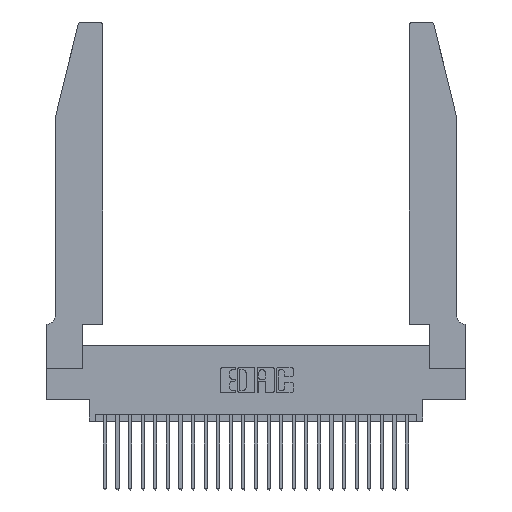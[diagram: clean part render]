
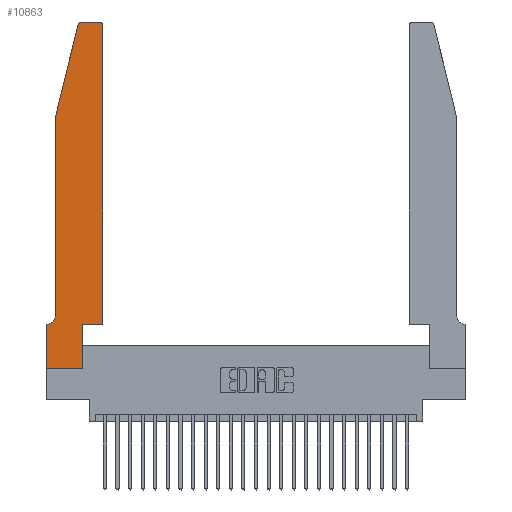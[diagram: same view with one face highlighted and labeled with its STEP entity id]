
A CAD part, top view. The second image highlights one B-rep face of the part: STEP entity #10863.
In plain terms, the highlighted planar face has unit normal (0, 0, 1).
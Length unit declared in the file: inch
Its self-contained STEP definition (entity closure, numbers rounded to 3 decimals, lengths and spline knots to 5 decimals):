
#157 = VERTEX_POINT ( 'NONE', #16407 ) ;
#285 = VECTOR ( 'NONE', #8463, 39.37008 ) ;
#910 = CIRCLE ( 'NONE', #12927, 0.03 ) ;
#916 = VERTEX_POINT ( 'NONE', #26282 ) ;
#1089 = LINE ( 'NONE', #9641, #23733 ) ;
#1887 = EDGE_CURVE ( 'NONE', #157, #13889, #9373, .T. ) ;
#2036 = VERTEX_POINT ( 'NONE', #17268 ) ;
#2094 = CARTESIAN_POINT ( 'NONE',  ( 0.284, 2.72, 0.37 ) ) ;
#2252 = CARTESIAN_POINT ( 'NONE',  ( 0.2865, 0.35, 0.37 ) ) ;
#2942 = ORIENTED_EDGE ( 'NONE', *, *, #4975, .T. ) ;
#3095 = CARTESIAN_POINT ( 'NONE',  ( 0.2605, 2.75, 0.37 ) ) ;
#3491 = CARTESIAN_POINT ( 'NONE',  ( 0.0755, 2., 0.37 ) ) ;
#3635 = ORIENTED_EDGE ( 'NONE', *, *, #1887, .T. ) ;
#3643 = CARTESIAN_POINT ( 'NONE',  ( 0.2865, 0.35, 0.37 ) ) ;
#3663 = VECTOR ( 'NONE', #6181, 39.37008 ) ;
#3993 = VERTEX_POINT ( 'NONE', #17073 ) ;
#4224 = CARTESIAN_POINT ( 'NONE',  ( 0., 0., 0.37 ) ) ;
#4352 = EDGE_CURVE ( 'NONE', #10704, #9987, #6673, .T. ) ;
#4615 = VERTEX_POINT ( 'NONE', #3491 ) ;
#4753 = DIRECTION ( 'NONE',  ( 1., 0., 0. ) ) ;
#4808 = DIRECTION ( 'NONE',  ( 1., 0., 0. ) ) ;
#4975 = EDGE_CURVE ( 'NONE', #25840, #17208, #22761, .T. ) ;
#5044 = VECTOR ( 'NONE', #5549, 39.37008 ) ;
#5361 = ORIENTED_EDGE ( 'NONE', *, *, #22117, .T. ) ;
#5549 = DIRECTION ( 'NONE',  ( 0., -1., 0. ) ) ;
#6181 = DIRECTION ( 'NONE',  ( 0., 1., 0. ) ) ;
#6673 = LINE ( 'NONE', #3095, #12470 ) ;
#7152 = LINE ( 'NONE', #15233, #22355 ) ;
#7387 = DIRECTION ( 'NONE',  ( -1., 0., 0. ) ) ;
#7452 = DIRECTION ( 'NONE',  ( -1., 0., 0. ) ) ;
#7631 = VECTOR ( 'NONE', #16535, 39.37008 ) ;
#7964 = CIRCLE ( 'NONE', #21372, 0.03 ) ;
#8151 = DIRECTION ( 'NONE',  ( -0.239, -0.971, 0. ) ) ;
#8463 = DIRECTION ( 'NONE',  ( 0., 1., 0. ) ) ;
#8710 = CARTESIAN_POINT ( 'NONE',  ( 0.4505, 2.72, 0.37 ) ) ;
#9137 = EDGE_CURVE ( 'NONE', #3993, #157, #12475, .T. ) ;
#9197 = ORIENTED_EDGE ( 'NONE', *, *, #24681, .T. ) ;
#9373 = LINE ( 'NONE', #2252, #285 ) ;
#9641 = CARTESIAN_POINT ( 'NONE',  ( 0.0755, 0.35, 0.37 ) ) ;
#9942 = CARTESIAN_POINT ( 'NONE',  ( 0.284, 2.75, 0.37 ) ) ;
#9987 = VERTEX_POINT ( 'NONE', #9942 ) ;
#10704 = VERTEX_POINT ( 'NONE', #20149 ) ;
#10863 = ADVANCED_FACE ( 'NONE', ( #24377 ), #24556, .T. ) ;
#11103 = ORIENTED_EDGE ( 'NONE', *, *, #12768, .T. ) ;
#11182 = VECTOR ( 'NONE', #4753, 39.37008 ) ;
#12092 = VECTOR ( 'NONE', #8151, 39.37008 ) ;
#12470 = VECTOR ( 'NONE', #7452, 39.37008 ) ;
#12475 = LINE ( 'NONE', #4224, #7631 ) ;
#12737 = LINE ( 'NONE', #14265, #12092 ) ;
#12768 = EDGE_CURVE ( 'NONE', #13889, #25840, #21846, .T. ) ;
#12797 = DIRECTION ( 'NONE',  ( 0., 0., -1. ) ) ;
#12927 = AXIS2_PLACEMENT_3D ( 'NONE', #2094, #18636, #26646 ) ;
#12943 = EDGE_CURVE ( 'NONE', #17208, #10704, #7964, .T. ) ;
#13015 = EDGE_CURVE ( 'NONE', #13371, #916, #1089, .T. ) ;
#13371 = VERTEX_POINT ( 'NONE', #23317 ) ;
#13590 = CARTESIAN_POINT ( 'NONE',  ( 0., 0., 0.37 ) ) ;
#13889 = VERTEX_POINT ( 'NONE', #3643 ) ;
#14265 = CARTESIAN_POINT ( 'NONE',  ( 0.0755, 2., 0.37 ) ) ;
#14547 = CARTESIAN_POINT ( 'NONE',  ( 0.4505, 0.35, 0.37 ) ) ;
#14853 = CARTESIAN_POINT ( 'NONE',  ( 0.0755, 0.42, 0.37 ) ) ;
#14884 = DIRECTION ( 'NONE',  ( -1., 0., 0. ) ) ;
#15233 = CARTESIAN_POINT ( 'NONE',  ( 0.0755, 2., 0.37 ) ) ;
#15401 = ORIENTED_EDGE ( 'NONE', *, *, #9137, .T. ) ;
#15583 = EDGE_LOOP ( 'NONE', ( #19989, #9197, #18039, #16935, #5361, #16533, #25935, #15401, #3635, #11103, #2942, #16297 ) ) ;
#15962 = CIRCLE ( 'NONE', #23748, 0.07 ) ;
#16040 = DIRECTION ( 'NONE',  ( 0., 0., 1. ) ) ;
#16297 = ORIENTED_EDGE ( 'NONE', *, *, #12943, .T. ) ;
#16407 = CARTESIAN_POINT ( 'NONE',  ( 0.2865, 0., 0.37 ) ) ;
#16533 = ORIENTED_EDGE ( 'NONE', *, *, #13015, .T. ) ;
#16535 = DIRECTION ( 'NONE',  ( 1., 0., 0. ) ) ;
#16935 = ORIENTED_EDGE ( 'NONE', *, *, #23853, .T. ) ;
#17073 = CARTESIAN_POINT ( 'NONE',  ( 0., 0., 0.37 ) ) ;
#17208 = VERTEX_POINT ( 'NONE', #8710 ) ;
#17268 = CARTESIAN_POINT ( 'NONE',  ( 0.25487, 2.72718, 0.37 ) ) ;
#18004 = LINE ( 'NONE', #13590, #5044 ) ;
#18039 = ORIENTED_EDGE ( 'NONE', *, *, #21970, .T. ) ;
#18432 = EDGE_CURVE ( 'NONE', #916, #3993, #18004, .T. ) ;
#18636 = DIRECTION ( 'NONE',  ( 0., 0., 1. ) ) ;
#19762 = AXIS2_PLACEMENT_3D ( 'NONE', #22205, #16040, #26280 ) ;
#19989 = ORIENTED_EDGE ( 'NONE', *, *, #4352, .T. ) ;
#20149 = CARTESIAN_POINT ( 'NONE',  ( 0.4205, 2.75, 0.37 ) ) ;
#21021 = CARTESIAN_POINT ( 'NONE',  ( 0.0055, 0.42, 0.37 ) ) ;
#21221 = CARTESIAN_POINT ( 'NONE',  ( 0.4505, 0.35, 0.37 ) ) ;
#21327 = CARTESIAN_POINT ( 'NONE',  ( 0.4205, 2.72, 0.37 ) ) ;
#21372 = AXIS2_PLACEMENT_3D ( 'NONE', #21327, #25449, #4808 ) ;
#21480 = DIRECTION ( 'NONE',  ( 0., -1., 0. ) ) ;
#21846 = LINE ( 'NONE', #21221, #11182 ) ;
#21970 = EDGE_CURVE ( 'NONE', #2036, #4615, #12737, .T. ) ;
#22117 = EDGE_CURVE ( 'NONE', #22859, #13371, #15962, .T. ) ;
#22205 = CARTESIAN_POINT ( 'NONE',  ( 0., 0.35, 0.37 ) ) ;
#22355 = VECTOR ( 'NONE', #21480, 39.37008 ) ;
#22761 = LINE ( 'NONE', #24711, #3663 ) ;
#22859 = VERTEX_POINT ( 'NONE', #14853 ) ;
#23317 = CARTESIAN_POINT ( 'NONE',  ( 0.0055, 0.35, 0.37 ) ) ;
#23733 = VECTOR ( 'NONE', #7387, 39.37008 ) ;
#23748 = AXIS2_PLACEMENT_3D ( 'NONE', #21021, #12797, #14884 ) ;
#23853 = EDGE_CURVE ( 'NONE', #4615, #22859, #7152, .T. ) ;
#24377 = FACE_OUTER_BOUND ( 'NONE', #15583, .T. ) ;
#24556 = PLANE ( 'NONE',  #19762 ) ;
#24681 = EDGE_CURVE ( 'NONE', #9987, #2036, #910, .T. ) ;
#24711 = CARTESIAN_POINT ( 'NONE',  ( 0.4505, 0.35, 0.37 ) ) ;
#25449 = DIRECTION ( 'NONE',  ( 0., 0., 1. ) ) ;
#25840 = VERTEX_POINT ( 'NONE', #14547 ) ;
#25935 = ORIENTED_EDGE ( 'NONE', *, *, #18432, .T. ) ;
#26280 = DIRECTION ( 'NONE',  ( 1., 0., 0. ) ) ;
#26282 = CARTESIAN_POINT ( 'NONE',  ( 0., 0.35, 0.37 ) ) ;
#26646 = DIRECTION ( 'NONE',  ( 1., 0., 0. ) ) ;
